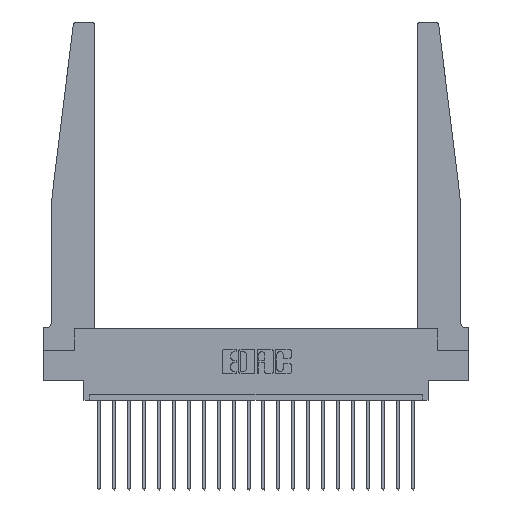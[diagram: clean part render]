
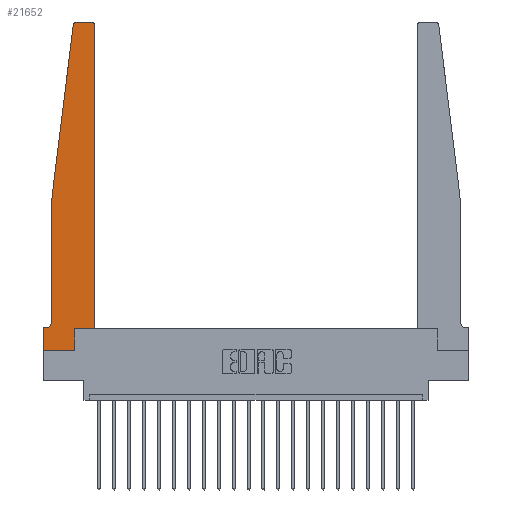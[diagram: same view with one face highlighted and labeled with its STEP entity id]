
A CAD part, top view. The second image highlights one B-rep face of the part: STEP entity #21652.
In plain terms, the highlighted planar face has unit normal (0, 0, 1).
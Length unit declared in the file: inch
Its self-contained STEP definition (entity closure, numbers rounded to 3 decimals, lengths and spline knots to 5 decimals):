
#170 = ORIENTED_EDGE ( 'NONE', *, *, #4085, .T. ) ;
#185 = VECTOR ( 'NONE', #16576, 39.37008 ) ;
#542 = ORIENTED_EDGE ( 'NONE', *, *, #15852, .T. ) ;
#662 = DIRECTION ( 'NONE',  ( 0., 1., 0. ) ) ;
#1205 = DIRECTION ( 'NONE',  ( -1., 0., 0. ) ) ;
#1221 = LINE ( 'NONE', #21112, #21639 ) ;
#1496 = CARTESIAN_POINT ( 'NONE',  ( 0.065, 1.25, 0.37 ) ) ;
#1593 = DIRECTION ( 'NONE',  ( 0., 0., 1. ) ) ;
#1607 = ORIENTED_EDGE ( 'NONE', *, *, #19175, .T. ) ;
#1645 = VERTEX_POINT ( 'NONE', #11992 ) ;
#1647 = CARTESIAN_POINT ( 'NONE',  ( 0.065, 0.2375, 0.37 ) ) ;
#1741 = EDGE_CURVE ( 'NONE', #5908, #19643, #8832, .T. ) ;
#2064 = VECTOR ( 'NONE', #4012, 39.37008 ) ;
#2282 = CARTESIAN_POINT ( 'NONE',  ( 0.2605, 0.18, 0.37 ) ) ;
#2334 = LINE ( 'NONE', #16046, #13747 ) ;
#2627 = AXIS2_PLACEMENT_3D ( 'NONE', #13170, #9885, #1205 ) ;
#3185 = ORIENTED_EDGE ( 'NONE', *, *, #13068, .T. ) ;
#3457 = VERTEX_POINT ( 'NONE', #6984 ) ;
#3598 = EDGE_CURVE ( 'NONE', #15944, #16503, #3903, .T. ) ;
#3695 = VECTOR ( 'NONE', #6581, 39.37008 ) ;
#3735 = VERTEX_POINT ( 'NONE', #1647 ) ;
#3903 = LINE ( 'NONE', #9167, #9169 ) ;
#3938 = LINE ( 'NONE', #5251, #4590 ) ;
#4012 = DIRECTION ( 'NONE',  ( 1., 0., 0. ) ) ;
#4085 = EDGE_CURVE ( 'NONE', #1645, #15764, #11620, .T. ) ;
#4190 = LINE ( 'NONE', #7482, #19181 ) ;
#4211 = VERTEX_POINT ( 'NONE', #13768 ) ;
#4286 = EDGE_CURVE ( 'NONE', #3457, #18462, #3938, .T. ) ;
#4590 = VECTOR ( 'NONE', #12245, 39.37008 ) ;
#4830 = CARTESIAN_POINT ( 'NONE',  ( 0., 0., 0.37 ) ) ;
#4990 = ORIENTED_EDGE ( 'NONE', *, *, #3598, .T. ) ;
#5251 = CARTESIAN_POINT ( 'NONE',  ( 0., 0., 0.37 ) ) ;
#5375 = VERTEX_POINT ( 'NONE', #10320 ) ;
#5783 = CARTESIAN_POINT ( 'NONE',  ( 0., 0.1875, 0.37 ) ) ;
#5861 = DIRECTION ( 'NONE',  ( 1., 0., 0. ) ) ;
#5908 = VERTEX_POINT ( 'NONE', #2282 ) ;
#6078 = DIRECTION ( 'NONE',  ( 0., 0., 1. ) ) ;
#6573 = CARTESIAN_POINT ( 'NONE',  ( 0.395, 2.72, 0.37 ) ) ;
#6581 = DIRECTION ( 'NONE',  ( 0., -1., 0. ) ) ;
#6685 = ORIENTED_EDGE ( 'NONE', *, *, #15750, .T. ) ;
#6984 = CARTESIAN_POINT ( 'NONE',  ( 0., 0., 0.37 ) ) ;
#7482 = CARTESIAN_POINT ( 'NONE',  ( 0.2605, 0.18, 0.37 ) ) ;
#7711 = EDGE_LOOP ( 'NONE', ( #170, #11808, #4990, #3185, #542, #1607, #21427, #14268, #6685, #20932, #16908, #15418 ) ) ;
#8425 = EDGE_CURVE ( 'NONE', #16741, #3457, #19432, .T. ) ;
#8832 = LINE ( 'NONE', #12321, #2064 ) ;
#9167 = CARTESIAN_POINT ( 'NONE',  ( 0.065, 1.25, 0.37 ) ) ;
#9169 = VECTOR ( 'NONE', #16369, 39.37008 ) ;
#9239 = AXIS2_PLACEMENT_3D ( 'NONE', #6573, #1593, #11803 ) ;
#9885 = DIRECTION ( 'NONE',  ( 0., 0., -1. ) ) ;
#10320 = CARTESIAN_POINT ( 'NONE',  ( 0.015, 0.1875, 0.37 ) ) ;
#10556 = VECTOR ( 'NONE', #16447, 39.37008 ) ;
#10711 = FACE_OUTER_BOUND ( 'NONE', #7711, .T. ) ;
#11005 = DIRECTION ( 'NONE',  ( 0., -1., 0. ) ) ;
#11620 = LINE ( 'NONE', #15104, #10556 ) ;
#11729 = CIRCLE ( 'NONE', #2627, 0.05 ) ;
#11803 = DIRECTION ( 'NONE',  ( 1., 0., 0. ) ) ;
#11808 = ORIENTED_EDGE ( 'NONE', *, *, #19279, .T. ) ;
#11992 = CARTESIAN_POINT ( 'NONE',  ( 0.395, 2.75, 0.37 ) ) ;
#12245 = DIRECTION ( 'NONE',  ( 1., 0., 0. ) ) ;
#12321 = CARTESIAN_POINT ( 'NONE',  ( 0.425, 0.18, 0.37 ) ) ;
#12542 = DIRECTION ( 'NONE',  ( -1., 0., 0. ) ) ;
#13068 = EDGE_CURVE ( 'NONE', #16503, #3735, #1221, .T. ) ;
#13094 = AXIS2_PLACEMENT_3D ( 'NONE', #20887, #6078, #5861 ) ;
#13170 = CARTESIAN_POINT ( 'NONE',  ( 0.015, 0.2375, 0.37 ) ) ;
#13747 = VECTOR ( 'NONE', #12542, 39.37008 ) ;
#13768 = CARTESIAN_POINT ( 'NONE',  ( 0.425, 2.72, 0.37 ) ) ;
#14137 = CARTESIAN_POINT ( 'NONE',  ( 0.27653, 2.75, 0.37 ) ) ;
#14268 = ORIENTED_EDGE ( 'NONE', *, *, #4286, .T. ) ;
#14321 = PLANE ( 'NONE',  #20547 ) ;
#14778 = CARTESIAN_POINT ( 'NONE',  ( 0.2605, 0., 0.37 ) ) ;
#14947 = CARTESIAN_POINT ( 'NONE',  ( 0., 0.1875, 0.37 ) ) ;
#15104 = CARTESIAN_POINT ( 'NONE',  ( 0.25, 2.75, 0.37 ) ) ;
#15418 = ORIENTED_EDGE ( 'NONE', *, *, #18523, .T. ) ;
#15748 = DIRECTION ( 'NONE',  ( 0., 0., 1. ) ) ;
#15750 = EDGE_CURVE ( 'NONE', #18462, #5908, #4190, .T. ) ;
#15764 = VERTEX_POINT ( 'NONE', #14137 ) ;
#15852 = EDGE_CURVE ( 'NONE', #3735, #5375, #11729, .T. ) ;
#15944 = VERTEX_POINT ( 'NONE', #17780 ) ;
#16024 = CARTESIAN_POINT ( 'NONE',  ( 0.425, 0.18, 0.37 ) ) ;
#16046 = CARTESIAN_POINT ( 'NONE',  ( 0.065, 0.1875, 0.37 ) ) ;
#16369 = DIRECTION ( 'NONE',  ( -0.122, -0.992, 0. ) ) ;
#16447 = DIRECTION ( 'NONE',  ( -1., 0., 0. ) ) ;
#16503 = VERTEX_POINT ( 'NONE', #1496 ) ;
#16576 = DIRECTION ( 'NONE',  ( 0., 1., 0. ) ) ;
#16741 = VERTEX_POINT ( 'NONE', #14947 ) ;
#16908 = ORIENTED_EDGE ( 'NONE', *, *, #21464, .T. ) ;
#17060 = CARTESIAN_POINT ( 'NONE',  ( 0.425, 0.18, 0.37 ) ) ;
#17780 = CARTESIAN_POINT ( 'NONE',  ( 0.24675, 2.72367, 0.37 ) ) ;
#18462 = VERTEX_POINT ( 'NONE', #14778 ) ;
#18523 = EDGE_CURVE ( 'NONE', #4211, #1645, #19034, .T. ) ;
#19034 = CIRCLE ( 'NONE', #9239, 0.03 ) ;
#19175 = EDGE_CURVE ( 'NONE', #5375, #16741, #2334, .T. ) ;
#19181 = VECTOR ( 'NONE', #662, 39.37008 ) ;
#19279 = EDGE_CURVE ( 'NONE', #15764, #15944, #21166, .T. ) ;
#19432 = LINE ( 'NONE', #4830, #3695 ) ;
#19643 = VERTEX_POINT ( 'NONE', #16024 ) ;
#20397 = LINE ( 'NONE', #17060, #185 ) ;
#20547 = AXIS2_PLACEMENT_3D ( 'NONE', #5783, #15748, #21044 ) ;
#20887 = CARTESIAN_POINT ( 'NONE',  ( 0.27653, 2.72, 0.37 ) ) ;
#20932 = ORIENTED_EDGE ( 'NONE', *, *, #1741, .T. ) ;
#21044 = DIRECTION ( 'NONE',  ( 1., 0., 0. ) ) ;
#21112 = CARTESIAN_POINT ( 'NONE',  ( 0.065, 1.25, 0.37 ) ) ;
#21166 = CIRCLE ( 'NONE', #13094, 0.03 ) ;
#21427 = ORIENTED_EDGE ( 'NONE', *, *, #8425, .T. ) ;
#21464 = EDGE_CURVE ( 'NONE', #19643, #4211, #20397, .T. ) ;
#21639 = VECTOR ( 'NONE', #11005, 39.37008 ) ;
#21652 = ADVANCED_FACE ( 'NONE', ( #10711 ), #14321, .T. ) ;
